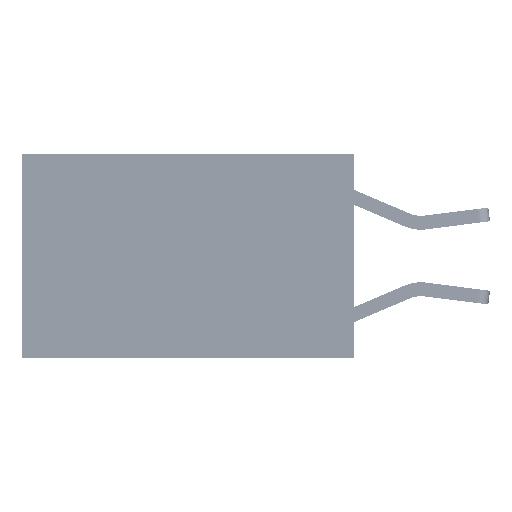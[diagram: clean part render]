
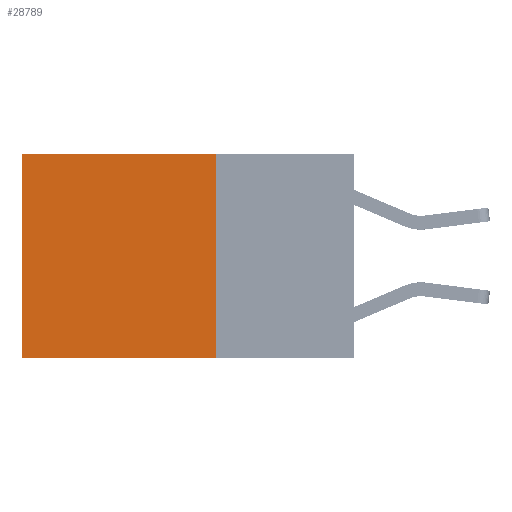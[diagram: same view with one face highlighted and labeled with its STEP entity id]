
A CAD part, left-side view. The second image highlights one B-rep face of the part: STEP entity #28789.
In plain terms, the highlighted planar face has unit normal (-1, 0, 0).
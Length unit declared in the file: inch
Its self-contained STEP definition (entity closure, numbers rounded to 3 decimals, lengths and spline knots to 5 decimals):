
#725 = VECTOR ( 'NONE', #13003, 39.37008 ) ;
#840 = VECTOR ( 'NONE', #9175, 39.37008 ) ;
#3126 = AXIS2_PLACEMENT_3D ( 'NONE', #3485, #23294, #8637 ) ;
#3485 = CARTESIAN_POINT ( 'NONE',  ( 0.2625, 0.25, 0. ) ) ;
#3839 = VERTEX_POINT ( 'NONE', #31162 ) ;
#5236 = CARTESIAN_POINT ( 'NONE',  ( 0.2625, 0.25, 0. ) ) ;
#5617 = CARTESIAN_POINT ( 'NONE',  ( 0.2625, 0.25, -0.37 ) ) ;
#5657 = VECTOR ( 'NONE', #14174, 39.37008 ) ;
#6104 = PLANE ( 'NONE',  #3126 ) ;
#6138 = EDGE_CURVE ( 'NONE', #3839, #27269, #13903, .T. ) ;
#6639 = ORIENTED_EDGE ( 'NONE', *, *, #15256, .T. ) ;
#7207 = EDGE_LOOP ( 'NONE', ( #13456, #18915, #14494, #6639 ) ) ;
#7977 = CARTESIAN_POINT ( 'NONE',  ( 0.2625, 0.6, -0.37 ) ) ;
#8051 = LINE ( 'NONE', #17921, #14555 ) ;
#8637 = DIRECTION ( 'NONE',  ( 0., 0., -1. ) ) ;
#9175 = DIRECTION ( 'NONE',  ( 0., 1., 0. ) ) ;
#10559 = CARTESIAN_POINT ( 'NONE',  ( 0.2625, 0.6, 0. ) ) ;
#13003 = DIRECTION ( 'NONE',  ( 0., 0., -1. ) ) ;
#13456 = ORIENTED_EDGE ( 'NONE', *, *, #6138, .T. ) ;
#13903 = LINE ( 'NONE', #10559, #725 ) ;
#14005 = CARTESIAN_POINT ( 'NONE',  ( 0.2625, 0.25, -0.37 ) ) ;
#14174 = DIRECTION ( 'NONE',  ( 0., 1., 0. ) ) ;
#14494 = ORIENTED_EDGE ( 'NONE', *, *, #24291, .F. ) ;
#14555 = VECTOR ( 'NONE', #20420, 39.37008 ) ;
#15256 = EDGE_CURVE ( 'NONE', #28573, #3839, #18787, .T. ) ;
#15513 = VERTEX_POINT ( 'NONE', #5617 ) ;
#17921 = CARTESIAN_POINT ( 'NONE',  ( 0.2625, 0.25, 0. ) ) ;
#18112 = FACE_OUTER_BOUND ( 'NONE', #7207, .T. ) ;
#18787 = LINE ( 'NONE', #31313, #5657 ) ;
#18915 = ORIENTED_EDGE ( 'NONE', *, *, #26339, .F. ) ;
#20420 = DIRECTION ( 'NONE',  ( 0., 0., -1. ) ) ;
#21348 = LINE ( 'NONE', #14005, #840 ) ;
#23294 = DIRECTION ( 'NONE',  ( 1., 0., 0. ) ) ;
#24291 = EDGE_CURVE ( 'NONE', #28573, #15513, #8051, .T. ) ;
#26339 = EDGE_CURVE ( 'NONE', #15513, #27269, #21348, .T. ) ;
#27269 = VERTEX_POINT ( 'NONE', #7977 ) ;
#28573 = VERTEX_POINT ( 'NONE', #5236 ) ;
#28789 = ADVANCED_FACE ( 'NONE', ( #18112 ), #6104, .F. ) ;
#31162 = CARTESIAN_POINT ( 'NONE',  ( 0.2625, 0.6, 0. ) ) ;
#31313 = CARTESIAN_POINT ( 'NONE',  ( 0.2625, 0.25, 0. ) ) ;
